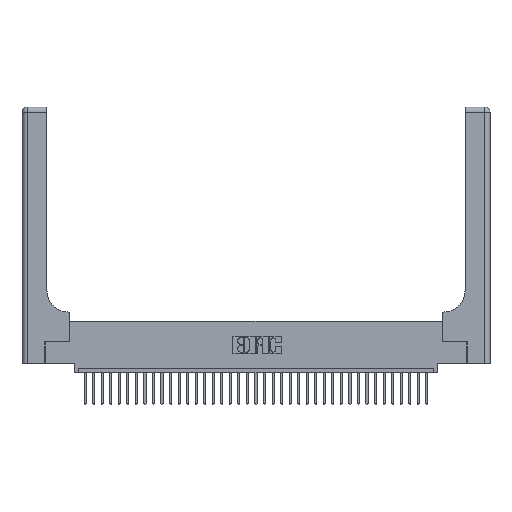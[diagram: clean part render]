
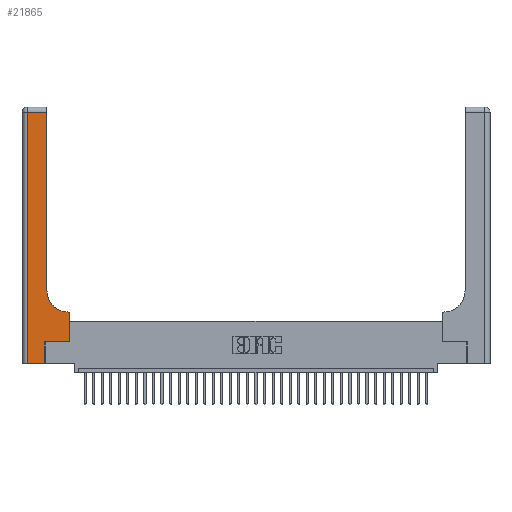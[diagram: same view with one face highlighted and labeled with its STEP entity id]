
A CAD part, top view. The second image highlights one B-rep face of the part: STEP entity #21865.
In plain terms, the highlighted planar face has unit normal (0, 0, 1).
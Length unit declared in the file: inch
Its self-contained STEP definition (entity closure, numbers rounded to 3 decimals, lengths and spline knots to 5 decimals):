
#196 = LINE ( 'NONE', #36196, #8522 ) ;
#812 = LINE ( 'NONE', #3320, #9189 ) ;
#1720 = FACE_OUTER_BOUND ( 'NONE', #33803, .T. ) ;
#2210 = DIRECTION ( 'NONE',  ( -1., 0., 0. ) ) ;
#2587 = DIRECTION ( 'NONE',  ( 0., 1., 0. ) ) ;
#3306 = ORIENTED_EDGE ( 'NONE', *, *, #23170, .T. ) ;
#3320 = CARTESIAN_POINT ( 'NONE',  ( 0.06, 3., 0.37 ) ) ;
#3379 = EDGE_CURVE ( 'NONE', #16204, #22490, #29919, .T. ) ;
#4727 = LINE ( 'NONE', #35810, #25415 ) ;
#6345 = CARTESIAN_POINT ( 'NONE',  ( 0.5585, 0.25, 0.37 ) ) ;
#7218 = LINE ( 'NONE', #6345, #8104 ) ;
#7263 = DIRECTION ( 'NONE',  ( 0., 0., -1. ) ) ;
#7483 = DIRECTION ( 'NONE',  ( 1., 0., 0. ) ) ;
#7749 = CARTESIAN_POINT ( 'NONE',  ( 0., 2.94, 0.37 ) ) ;
#7998 = EDGE_CURVE ( 'NONE', #25982, #34511, #21732, .T. ) ;
#8104 = VECTOR ( 'NONE', #31127, 39.37008 ) ;
#8522 = VECTOR ( 'NONE', #2587, 39.37008 ) ;
#9146 = VERTEX_POINT ( 'NONE', #13296 ) ;
#9189 = VECTOR ( 'NONE', #34221, 39.37008 ) ;
#9779 = VERTEX_POINT ( 'NONE', #25006 ) ;
#10670 = VERTEX_POINT ( 'NONE', #19244 ) ;
#11815 = CARTESIAN_POINT ( 'NONE',  ( 0., 3., 0.37 ) ) ;
#12187 = ORIENTED_EDGE ( 'NONE', *, *, #25467, .T. ) ;
#13296 = CARTESIAN_POINT ( 'NONE',  ( 0.5585, 0.25, 0.37 ) ) ;
#13794 = ORIENTED_EDGE ( 'NONE', *, *, #22637, .T. ) ;
#13895 = ORIENTED_EDGE ( 'NONE', *, *, #25291, .T. ) ;
#14114 = CARTESIAN_POINT ( 'NONE',  ( 0., 0., 0.37 ) ) ;
#14475 = VECTOR ( 'NONE', #16166, 39.37008 ) ;
#14664 = DIRECTION ( 'NONE',  ( 0., 0., -1. ) ) ;
#16166 = DIRECTION ( 'NONE',  ( 0., 1., 0. ) ) ;
#16204 = VERTEX_POINT ( 'NONE', #31932 ) ;
#16680 = ORIENTED_EDGE ( 'NONE', *, *, #33700, .T. ) ;
#18534 = CARTESIAN_POINT ( 'NONE',  ( 0.269, 0., 0.37 ) ) ;
#19244 = CARTESIAN_POINT ( 'NONE',  ( 0.2915, 2.94, 0.37 ) ) ;
#19749 = VERTEX_POINT ( 'NONE', #34036 ) ;
#20339 = ORIENTED_EDGE ( 'NONE', *, *, #7998, .T. ) ;
#20638 = EDGE_CURVE ( 'NONE', #9779, #9146, #4727, .T. ) ;
#20818 = AXIS2_PLACEMENT_3D ( 'NONE', #21295, #7263, #32989 ) ;
#20954 = CARTESIAN_POINT ( 'NONE',  ( 0.5415, 0.6, 0.37 ) ) ;
#21295 = CARTESIAN_POINT ( 'NONE',  ( 0.5415, 0.85, 0.37 ) ) ;
#21732 = LINE ( 'NONE', #14114, #35714 ) ;
#21865 = ADVANCED_FACE ( 'NONE', ( #1720 ), #31390, .F. ) ;
#22490 = VERTEX_POINT ( 'NONE', #20954 ) ;
#22637 = EDGE_CURVE ( 'NONE', #27346, #10670, #36329, .T. ) ;
#23170 = EDGE_CURVE ( 'NONE', #22490, #27346, #30141, .T. ) ;
#25002 = AXIS2_PLACEMENT_3D ( 'NONE', #11815, #14664, #28621 ) ;
#25006 = CARTESIAN_POINT ( 'NONE',  ( 0.269, 0.25, 0.37 ) ) ;
#25130 = DIRECTION ( 'NONE',  ( 1., 0., 0. ) ) ;
#25291 = EDGE_CURVE ( 'NONE', #10670, #19749, #32195, .T. ) ;
#25415 = VECTOR ( 'NONE', #7483, 39.37008 ) ;
#25467 = EDGE_CURVE ( 'NONE', #34511, #9779, #196, .T. ) ;
#25982 = VERTEX_POINT ( 'NONE', #32724 ) ;
#26560 = VECTOR ( 'NONE', #2210, 39.37008 ) ;
#27303 = VECTOR ( 'NONE', #31958, 39.37008 ) ;
#27346 = VERTEX_POINT ( 'NONE', #30794 ) ;
#28621 = DIRECTION ( 'NONE',  ( -1., 0., 0. ) ) ;
#28642 = ORIENTED_EDGE ( 'NONE', *, *, #34262, .T. ) ;
#29162 = CARTESIAN_POINT ( 'NONE',  ( 0.2915, 0.6, 0.37 ) ) ;
#29744 = CARTESIAN_POINT ( 'NONE',  ( 0.2915, 3., 0.37 ) ) ;
#29919 = LINE ( 'NONE', #29162, #27303 ) ;
#30064 = ORIENTED_EDGE ( 'NONE', *, *, #3379, .T. ) ;
#30141 = CIRCLE ( 'NONE', #20818, 0.25 ) ;
#30794 = CARTESIAN_POINT ( 'NONE',  ( 0.2915, 0.85, 0.37 ) ) ;
#31048 = ORIENTED_EDGE ( 'NONE', *, *, #20638, .T. ) ;
#31127 = DIRECTION ( 'NONE',  ( 0., 1., 0. ) ) ;
#31390 = PLANE ( 'NONE',  #25002 ) ;
#31932 = CARTESIAN_POINT ( 'NONE',  ( 0.5585, 0.6, 0.37 ) ) ;
#31958 = DIRECTION ( 'NONE',  ( -1., 0., 0. ) ) ;
#32195 = LINE ( 'NONE', #7749, #26560 ) ;
#32724 = CARTESIAN_POINT ( 'NONE',  ( 0.06, 0., 0.37 ) ) ;
#32989 = DIRECTION ( 'NONE',  ( 1., 0., 0. ) ) ;
#33700 = EDGE_CURVE ( 'NONE', #19749, #25982, #812, .T. ) ;
#33803 = EDGE_LOOP ( 'NONE', ( #13794, #13895, #16680, #20339, #12187, #31048, #28642, #30064, #3306 ) ) ;
#34036 = CARTESIAN_POINT ( 'NONE',  ( 0.06, 2.94, 0.37 ) ) ;
#34221 = DIRECTION ( 'NONE',  ( 0., -1., 0. ) ) ;
#34262 = EDGE_CURVE ( 'NONE', #9146, #16204, #7218, .T. ) ;
#34511 = VERTEX_POINT ( 'NONE', #18534 ) ;
#35714 = VECTOR ( 'NONE', #25130, 39.37008 ) ;
#35810 = CARTESIAN_POINT ( 'NONE',  ( 0.269, 0.25, 0.37 ) ) ;
#36196 = CARTESIAN_POINT ( 'NONE',  ( 0.269, 0., 0.37 ) ) ;
#36329 = LINE ( 'NONE', #29744, #14475 ) ;
